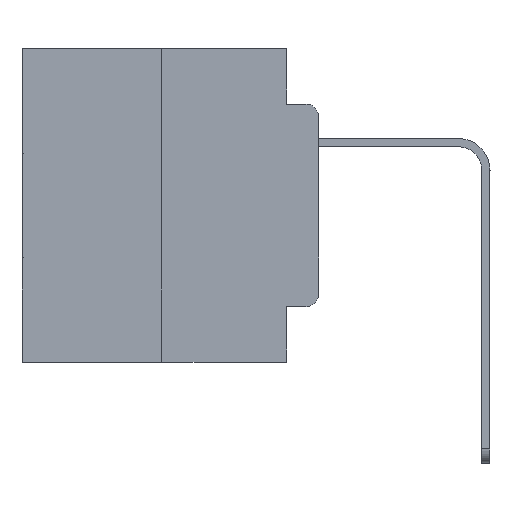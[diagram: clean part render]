
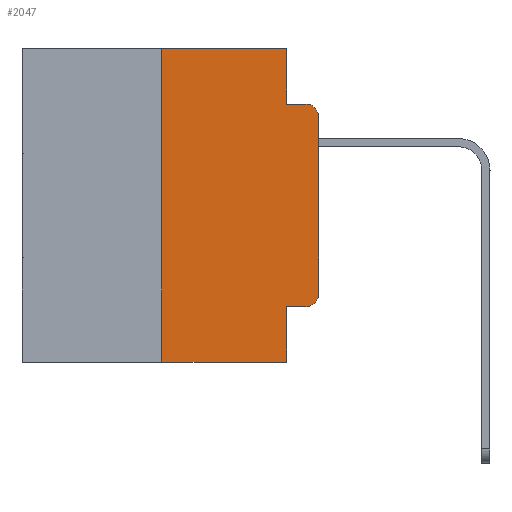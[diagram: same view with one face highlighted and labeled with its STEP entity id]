
A CAD part, left-side view. The second image highlights one B-rep face of the part: STEP entity #2047.
In plain terms, the highlighted planar face has unit normal (-1, 0, 0).
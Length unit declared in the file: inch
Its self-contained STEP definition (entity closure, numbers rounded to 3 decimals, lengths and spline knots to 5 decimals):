
#269 = DIRECTION ( 'NONE',  ( 0., -1., 0. ) ) ;
#863 = CARTESIAN_POINT ( 'NONE',  ( 0., 0.051, 0. ) ) ;
#925 = VECTOR ( 'NONE', #11279, 39.37008 ) ;
#1046 = ORIENTED_EDGE ( 'NONE', *, *, #23728, .F. ) ;
#1398 = ORIENTED_EDGE ( 'NONE', *, *, #3438, .F. ) ;
#2047 = ADVANCED_FACE ( 'NONE', ( #24152 ), #27418, .F. ) ;
#2064 = LINE ( 'NONE', #8068, #14765 ) ;
#2233 = CARTESIAN_POINT ( 'NONE',  ( 0., 0.051, 0. ) ) ;
#2465 = ORIENTED_EDGE ( 'NONE', *, *, #7825, .T. ) ;
#3341 = CARTESIAN_POINT ( 'NONE',  ( 0., 0.473, 0. ) ) ;
#3438 = EDGE_CURVE ( 'NONE', #11040, #7095, #28240, .T. ) ;
#4747 = ORIENTED_EDGE ( 'NONE', *, *, #19426, .F. ) ;
#5003 = VECTOR ( 'NONE', #21299, 39.37008 ) ;
#5328 = DIRECTION ( 'NONE',  ( 0., -1., 0. ) ) ;
#5725 = AXIS2_PLACEMENT_3D ( 'NONE', #15672, #26587, #20198 ) ;
#6140 = ORIENTED_EDGE ( 'NONE', *, *, #12801, .T. ) ;
#6207 = VERTEX_POINT ( 'NONE', #22145 ) ;
#6320 = EDGE_CURVE ( 'NONE', #22298, #6207, #7831, .T. ) ;
#6933 = VECTOR ( 'NONE', #5328, 39.37008 ) ;
#7095 = VERTEX_POINT ( 'NONE', #27533 ) ;
#7628 = LINE ( 'NONE', #9106, #10700 ) ;
#7657 = VECTOR ( 'NONE', #269, 39.37008 ) ;
#7825 = EDGE_CURVE ( 'NONE', #11040, #8941, #15980, .T. ) ;
#7831 = CIRCLE ( 'NONE', #13648, 0.02 ) ;
#7994 = DIRECTION ( 'NONE',  ( -1., 0., 0. ) ) ;
#8068 = CARTESIAN_POINT ( 'NONE',  ( 0., 0., 0. ) ) ;
#8204 = CARTESIAN_POINT ( 'NONE',  ( 0., 0.02, -0.4115 ) ) ;
#8941 = VERTEX_POINT ( 'NONE', #12328 ) ;
#9106 = CARTESIAN_POINT ( 'NONE',  ( 0., 0.051, 0. ) ) ;
#9811 = DIRECTION ( 'NONE',  ( 1., 0., 0. ) ) ;
#10193 = CARTESIAN_POINT ( 'NONE',  ( 0., 0.02, -0.3915 ) ) ;
#10409 = VERTEX_POINT ( 'NONE', #24705 ) ;
#10472 = VERTEX_POINT ( 'NONE', #27492 ) ;
#10700 = VECTOR ( 'NONE', #24470, 39.37008 ) ;
#11040 = VERTEX_POINT ( 'NONE', #24774 ) ;
#11229 = VERTEX_POINT ( 'NONE', #12835 ) ;
#11279 = DIRECTION ( 'NONE',  ( 0., 0., -1. ) ) ;
#11868 = CARTESIAN_POINT ( 'NONE',  ( 0., 0.473, 0. ) ) ;
#12111 = LINE ( 'NONE', #26564, #7657 ) ;
#12328 = CARTESIAN_POINT ( 'NONE',  ( 0., 0.051, -0.5 ) ) ;
#12801 = EDGE_CURVE ( 'NONE', #6207, #10409, #2064, .T. ) ;
#12835 = CARTESIAN_POINT ( 'NONE',  ( 0., 0.02, -0.0885 ) ) ;
#13530 = EDGE_CURVE ( 'NONE', #10409, #11229, #14082, .T. ) ;
#13648 = AXIS2_PLACEMENT_3D ( 'NONE', #10193, #7994, #23283 ) ;
#14082 = CIRCLE ( 'NONE', #5725, 0.02 ) ;
#14667 = CARTESIAN_POINT ( 'NONE',  ( 0., 0.473, -0.5 ) ) ;
#14765 = VECTOR ( 'NONE', #21278, 39.37008 ) ;
#14809 = CARTESIAN_POINT ( 'NONE',  ( 0., 0.25, 0. ) ) ;
#14899 = DIRECTION ( 'NONE',  ( 0., 0., 1. ) ) ;
#15035 = EDGE_LOOP ( 'NONE', ( #6140, #26378, #4747, #17518, #24756, #1398, #2465, #1046, #19244, #16517 ) ) ;
#15266 = VERTEX_POINT ( 'NONE', #863 ) ;
#15672 = CARTESIAN_POINT ( 'NONE',  ( 0., 0.02, -0.1085 ) ) ;
#15980 = LINE ( 'NONE', #14667, #5003 ) ;
#16395 = DIRECTION ( 'NONE',  ( 0., 0., -1. ) ) ;
#16517 = ORIENTED_EDGE ( 'NONE', *, *, #6320, .T. ) ;
#16590 = VECTOR ( 'NONE', #14899, 39.37008 ) ;
#17003 = CARTESIAN_POINT ( 'NONE',  ( 0., 0.051, -0.0885 ) ) ;
#17518 = ORIENTED_EDGE ( 'NONE', *, *, #27799, .F. ) ;
#18582 = VERTEX_POINT ( 'NONE', #21474 ) ;
#19047 = DIRECTION ( 'NONE',  ( 0., -1., 0. ) ) ;
#19244 = ORIENTED_EDGE ( 'NONE', *, *, #27046, .T. ) ;
#19426 = EDGE_CURVE ( 'NONE', #18582, #11229, #22106, .T. ) ;
#20198 = DIRECTION ( 'NONE',  ( 0., 0., -1. ) ) ;
#21278 = DIRECTION ( 'NONE',  ( 0., 0., 1. ) ) ;
#21299 = DIRECTION ( 'NONE',  ( 0., -1., 0. ) ) ;
#21474 = CARTESIAN_POINT ( 'NONE',  ( 0., 0.051, -0.0885 ) ) ;
#22008 = EDGE_CURVE ( 'NONE', #7095, #15266, #26800, .T. ) ;
#22106 = LINE ( 'NONE', #17003, #23467 ) ;
#22145 = CARTESIAN_POINT ( 'NONE',  ( 0., 0., -0.3915 ) ) ;
#22298 = VERTEX_POINT ( 'NONE', #8204 ) ;
#23283 = DIRECTION ( 'NONE',  ( 0., 0., -1. ) ) ;
#23467 = VECTOR ( 'NONE', #19047, 39.37008 ) ;
#23728 = EDGE_CURVE ( 'NONE', #10472, #8941, #25982, .T. ) ;
#24152 = FACE_OUTER_BOUND ( 'NONE', #15035, .T. ) ;
#24470 = DIRECTION ( 'NONE',  ( 0., 0., -1. ) ) ;
#24705 = CARTESIAN_POINT ( 'NONE',  ( 0., 0., -0.1085 ) ) ;
#24756 = ORIENTED_EDGE ( 'NONE', *, *, #22008, .F. ) ;
#24774 = CARTESIAN_POINT ( 'NONE',  ( 0., 0.25, -0.5 ) ) ;
#25590 = AXIS2_PLACEMENT_3D ( 'NONE', #3341, #9811, #16395 ) ;
#25982 = LINE ( 'NONE', #2233, #925 ) ;
#26378 = ORIENTED_EDGE ( 'NONE', *, *, #13530, .T. ) ;
#26564 = CARTESIAN_POINT ( 'NONE',  ( 0., 0.051, -0.4115 ) ) ;
#26587 = DIRECTION ( 'NONE',  ( -1., 0., 0. ) ) ;
#26800 = LINE ( 'NONE', #11868, #6933 ) ;
#27046 = EDGE_CURVE ( 'NONE', #10472, #22298, #12111, .T. ) ;
#27418 = PLANE ( 'NONE',  #25590 ) ;
#27492 = CARTESIAN_POINT ( 'NONE',  ( 0., 0.051, -0.4115 ) ) ;
#27533 = CARTESIAN_POINT ( 'NONE',  ( 0., 0.25, 0. ) ) ;
#27799 = EDGE_CURVE ( 'NONE', #15266, #18582, #7628, .T. ) ;
#28240 = LINE ( 'NONE', #14809, #16590 ) ;
